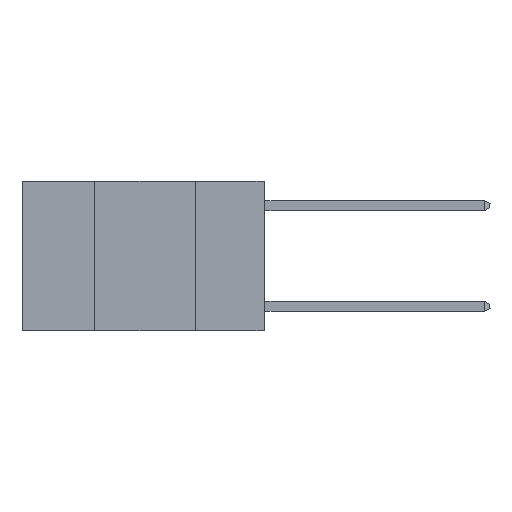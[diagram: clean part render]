
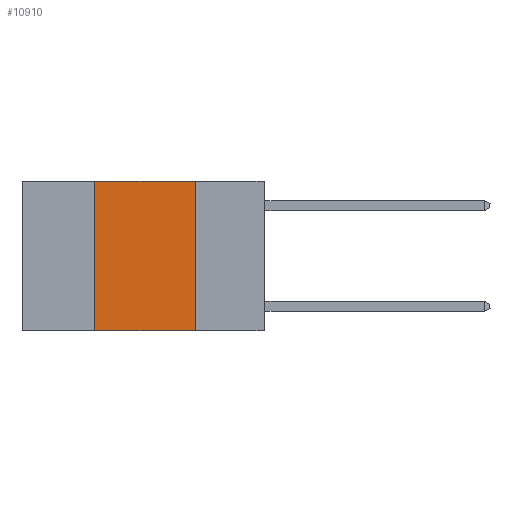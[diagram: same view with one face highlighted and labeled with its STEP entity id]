
A CAD part, left-side view. The second image highlights one B-rep face of the part: STEP entity #10910.
In plain terms, the highlighted planar face has unit normal (-1, 0, 0).
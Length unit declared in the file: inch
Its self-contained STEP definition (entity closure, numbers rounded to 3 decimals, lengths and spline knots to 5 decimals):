
#624 = EDGE_CURVE ( 'NONE', #7030, #21267, #6341, .T. ) ;
#709 = DIRECTION ( 'NONE',  ( 0., -1., 0. ) ) ;
#714 = EDGE_CURVE ( 'NONE', #7030, #11865, #13215, .T. ) ;
#1954 = ORIENTED_EDGE ( 'NONE', *, *, #13506, .F. ) ;
#2218 = DIRECTION ( 'NONE',  ( 0., 0., -1. ) ) ;
#3378 = DIRECTION ( 'NONE',  ( 0., 0., -1. ) ) ;
#4311 = CARTESIAN_POINT ( 'NONE',  ( 0., 0.6, -0.37 ) ) ;
#5122 = FACE_OUTER_BOUND ( 'NONE', #14208, .T. ) ;
#6341 = LINE ( 'NONE', #20580, #20688 ) ;
#7030 = VERTEX_POINT ( 'NONE', #16903 ) ;
#7601 = AXIS2_PLACEMENT_3D ( 'NONE', #21363, #22900, #3378 ) ;
#7821 = ORIENTED_EDGE ( 'NONE', *, *, #624, .F. ) ;
#7962 = LINE ( 'NONE', #22186, #13184 ) ;
#8480 = VECTOR ( 'NONE', #19977, 39.37008 ) ;
#9134 = LINE ( 'NONE', #11001, #8480 ) ;
#10910 = ADVANCED_FACE ( 'NONE', ( #5122 ), #14253, .F. ) ;
#11001 = CARTESIAN_POINT ( 'NONE',  ( 0., 0.6, 0. ) ) ;
#11708 = CARTESIAN_POINT ( 'NONE',  ( 0., 0.17, -0.37 ) ) ;
#11865 = VERTEX_POINT ( 'NONE', #11708 ) ;
#12229 = EDGE_CURVE ( 'NONE', #17934, #11865, #7962, .T. ) ;
#12326 = ORIENTED_EDGE ( 'NONE', *, *, #12229, .F. ) ;
#13184 = VECTOR ( 'NONE', #2218, 39.37008 ) ;
#13215 = LINE ( 'NONE', #4311, #15487 ) ;
#13506 = EDGE_CURVE ( 'NONE', #21267, #17934, #9134, .T. ) ;
#13757 = CARTESIAN_POINT ( 'NONE',  ( 0., 0.42, 0. ) ) ;
#14208 = EDGE_LOOP ( 'NONE', ( #12326, #1954, #7821, #21469 ) ) ;
#14253 = PLANE ( 'NONE',  #7601 ) ;
#15487 = VECTOR ( 'NONE', #709, 39.37008 ) ;
#16858 = DIRECTION ( 'NONE',  ( 0., 0., 1. ) ) ;
#16903 = CARTESIAN_POINT ( 'NONE',  ( 0., 0.42, -0.37 ) ) ;
#17934 = VERTEX_POINT ( 'NONE', #20314 ) ;
#19977 = DIRECTION ( 'NONE',  ( 0., -1., 0. ) ) ;
#20314 = CARTESIAN_POINT ( 'NONE',  ( 0., 0.17, 0. ) ) ;
#20580 = CARTESIAN_POINT ( 'NONE',  ( 0., 0.42, 0. ) ) ;
#20688 = VECTOR ( 'NONE', #16858, 39.37008 ) ;
#21267 = VERTEX_POINT ( 'NONE', #13757 ) ;
#21363 = CARTESIAN_POINT ( 'NONE',  ( 0., 0.6, 0. ) ) ;
#21469 = ORIENTED_EDGE ( 'NONE', *, *, #714, .T. ) ;
#22186 = CARTESIAN_POINT ( 'NONE',  ( 0., 0.17, 0. ) ) ;
#22900 = DIRECTION ( 'NONE',  ( 1., 0., 0. ) ) ;
